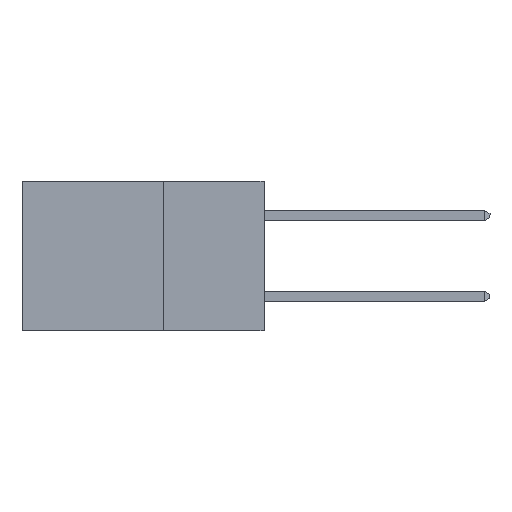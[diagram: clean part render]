
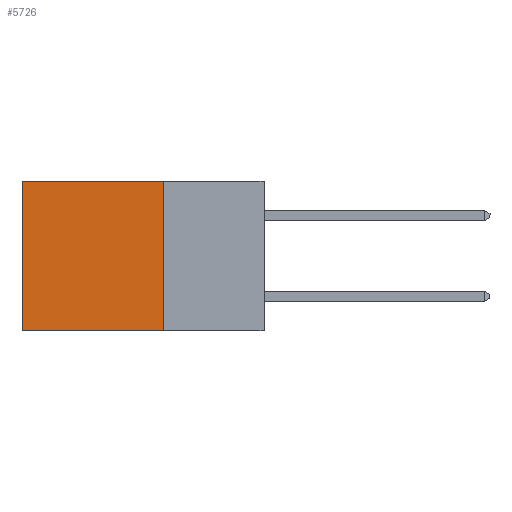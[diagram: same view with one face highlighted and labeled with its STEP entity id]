
A CAD part, left-side view. The second image highlights one B-rep face of the part: STEP entity #5726.
In plain terms, the highlighted planar face has unit normal (-1, 0, 0).
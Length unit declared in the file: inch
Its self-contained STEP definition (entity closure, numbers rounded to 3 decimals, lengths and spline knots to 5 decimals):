
#137 = ORIENTED_EDGE ( 'NONE', *, *, #10960, .T. ) ;
#687 = LINE ( 'NONE', #4408, #10158 ) ;
#742 = VECTOR ( 'NONE', #9342, 39.37008 ) ;
#1024 = EDGE_CURVE ( 'NONE', #1392, #9138, #687, .T. ) ;
#1032 = LINE ( 'NONE', #11741, #10467 ) ;
#1288 = EDGE_LOOP ( 'NONE', ( #137, #5051, #7450, #2947 ) ) ;
#1392 = VERTEX_POINT ( 'NONE', #3514 ) ;
#1606 = VECTOR ( 'NONE', #5905, 39.37008 ) ;
#2303 = AXIS2_PLACEMENT_3D ( 'NONE', #6916, #8768, #3335 ) ;
#2435 = PLANE ( 'NONE',  #2303 ) ;
#2947 = ORIENTED_EDGE ( 'NONE', *, *, #5527, .T. ) ;
#3335 = DIRECTION ( 'NONE',  ( 0., 0., -1. ) ) ;
#3514 = CARTESIAN_POINT ( 'NONE',  ( 0.298, 0.25, -0.37 ) ) ;
#4330 = LINE ( 'NONE', #5004, #1606 ) ;
#4408 = CARTESIAN_POINT ( 'NONE',  ( 0.298, 0.25, -0.37 ) ) ;
#4631 = VERTEX_POINT ( 'NONE', #10662 ) ;
#5004 = CARTESIAN_POINT ( 'NONE',  ( 0.298, 0.6, 0. ) ) ;
#5051 = ORIENTED_EDGE ( 'NONE', *, *, #1024, .F. ) ;
#5527 = EDGE_CURVE ( 'NONE', #6948, #4631, #5637, .T. ) ;
#5637 = LINE ( 'NONE', #5661, #742 ) ;
#5661 = CARTESIAN_POINT ( 'NONE',  ( 0.298, 0.25, 0. ) ) ;
#5726 = ADVANCED_FACE ( 'NONE', ( #10617 ), #2435, .F. ) ;
#5905 = DIRECTION ( 'NONE',  ( 0., 0., -1. ) ) ;
#5933 = EDGE_CURVE ( 'NONE', #6948, #1392, #1032, .T. ) ;
#6916 = CARTESIAN_POINT ( 'NONE',  ( 0.298, 0.25, 0. ) ) ;
#6948 = VERTEX_POINT ( 'NONE', #10832 ) ;
#7450 = ORIENTED_EDGE ( 'NONE', *, *, #5933, .F. ) ;
#7522 = CARTESIAN_POINT ( 'NONE',  ( 0.298, 0.6, -0.37 ) ) ;
#8173 = DIRECTION ( 'NONE',  ( 0., 0., -1. ) ) ;
#8768 = DIRECTION ( 'NONE',  ( 1., 0., 0. ) ) ;
#9138 = VERTEX_POINT ( 'NONE', #7522 ) ;
#9342 = DIRECTION ( 'NONE',  ( 0., 1., 0. ) ) ;
#10158 = VECTOR ( 'NONE', #11064, 39.37008 ) ;
#10467 = VECTOR ( 'NONE', #8173, 39.37008 ) ;
#10617 = FACE_OUTER_BOUND ( 'NONE', #1288, .T. ) ;
#10662 = CARTESIAN_POINT ( 'NONE',  ( 0.298, 0.6, 0. ) ) ;
#10832 = CARTESIAN_POINT ( 'NONE',  ( 0.298, 0.25, 0. ) ) ;
#10960 = EDGE_CURVE ( 'NONE', #4631, #9138, #4330, .T. ) ;
#11064 = DIRECTION ( 'NONE',  ( 0., 1., 0. ) ) ;
#11741 = CARTESIAN_POINT ( 'NONE',  ( 0.298, 0.25, 0. ) ) ;
